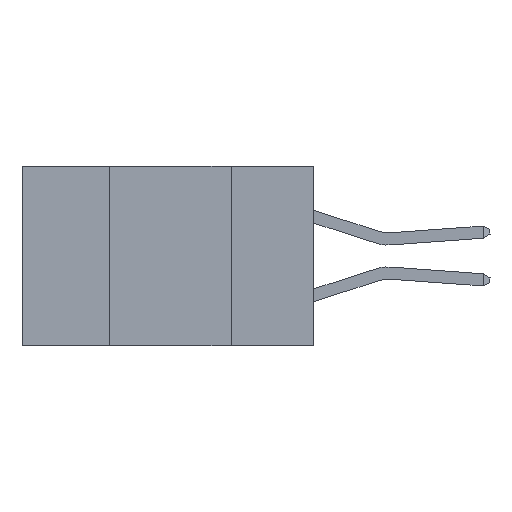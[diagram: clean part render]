
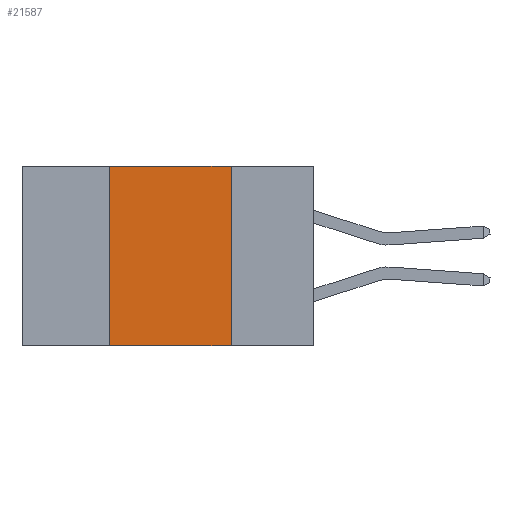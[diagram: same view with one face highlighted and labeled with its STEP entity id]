
A CAD part, left-side view. The second image highlights one B-rep face of the part: STEP entity #21587.
In plain terms, the highlighted planar face has unit normal (-1, 0, 0).
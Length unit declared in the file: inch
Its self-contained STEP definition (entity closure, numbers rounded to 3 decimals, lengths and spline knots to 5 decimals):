
#623 = AXIS2_PLACEMENT_3D ( 'NONE', #1199, #18332, #19856 ) ;
#889 = VERTEX_POINT ( 'NONE', #6762 ) ;
#1199 = CARTESIAN_POINT ( 'NONE',  ( 0., 0.6, 0. ) ) ;
#1953 = LINE ( 'NONE', #6408, #10454 ) ;
#2765 = PLANE ( 'NONE',  #623 ) ;
#2904 = DIRECTION ( 'NONE',  ( 0., -1., 0. ) ) ;
#4329 = DIRECTION ( 'NONE',  ( 0., -1., 0. ) ) ;
#4997 = LINE ( 'NONE', #8764, #13497 ) ;
#6408 = CARTESIAN_POINT ( 'NONE',  ( 0., 0.6, -0.37 ) ) ;
#6602 = ORIENTED_EDGE ( 'NONE', *, *, #21578, .T. ) ;
#6762 = CARTESIAN_POINT ( 'NONE',  ( 0., 0.17, 0. ) ) ;
#6908 = CARTESIAN_POINT ( 'NONE',  ( 0., 0.42, 0. ) ) ;
#8640 = LINE ( 'NONE', #12698, #16415 ) ;
#8764 = CARTESIAN_POINT ( 'NONE',  ( 0., 0.17, 0. ) ) ;
#9111 = ORIENTED_EDGE ( 'NONE', *, *, #15502, .F. ) ;
#10454 = VECTOR ( 'NONE', #2904, 39.37008 ) ;
#10991 = FACE_OUTER_BOUND ( 'NONE', #16851, .T. ) ;
#11014 = EDGE_CURVE ( 'NONE', #16286, #16011, #20864, .T. ) ;
#11789 = VECTOR ( 'NONE', #15747, 39.37008 ) ;
#12280 = CARTESIAN_POINT ( 'NONE',  ( 0., 0.42, 0. ) ) ;
#12698 = CARTESIAN_POINT ( 'NONE',  ( 0., 0.6, 0. ) ) ;
#12915 = ORIENTED_EDGE ( 'NONE', *, *, #11014, .F. ) ;
#13497 = VECTOR ( 'NONE', #17252, 39.37008 ) ;
#14594 = VERTEX_POINT ( 'NONE', #18193 ) ;
#15502 = EDGE_CURVE ( 'NONE', #889, #14594, #4997, .T. ) ;
#15747 = DIRECTION ( 'NONE',  ( 0., 0., 1. ) ) ;
#16003 = CARTESIAN_POINT ( 'NONE',  ( 0., 0.42, -0.37 ) ) ;
#16011 = VERTEX_POINT ( 'NONE', #6908 ) ;
#16286 = VERTEX_POINT ( 'NONE', #16003 ) ;
#16415 = VECTOR ( 'NONE', #4329, 39.37008 ) ;
#16851 = EDGE_LOOP ( 'NONE', ( #9111, #18688, #12915, #6602 ) ) ;
#17252 = DIRECTION ( 'NONE',  ( 0., 0., -1. ) ) ;
#18193 = CARTESIAN_POINT ( 'NONE',  ( 0., 0.17, -0.37 ) ) ;
#18332 = DIRECTION ( 'NONE',  ( 1., 0., 0. ) ) ;
#18688 = ORIENTED_EDGE ( 'NONE', *, *, #19532, .F. ) ;
#19532 = EDGE_CURVE ( 'NONE', #16011, #889, #8640, .T. ) ;
#19856 = DIRECTION ( 'NONE',  ( 0., 0., -1. ) ) ;
#20864 = LINE ( 'NONE', #12280, #11789 ) ;
#21578 = EDGE_CURVE ( 'NONE', #16286, #14594, #1953, .T. ) ;
#21587 = ADVANCED_FACE ( 'NONE', ( #10991 ), #2765, .F. ) ;
